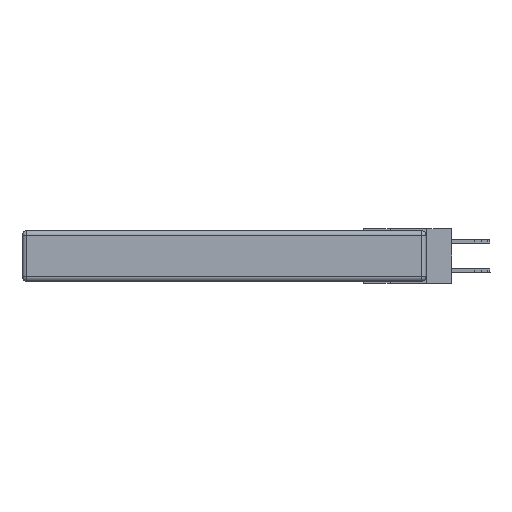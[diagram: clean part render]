
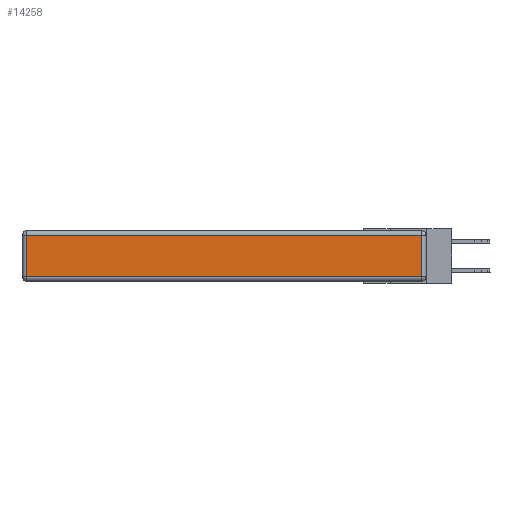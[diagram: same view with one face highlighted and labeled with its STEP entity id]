
A CAD part, left-side view. The second image highlights one B-rep face of the part: STEP entity #14258.
In plain terms, the highlighted planar face has unit normal (-1, 0, 0).
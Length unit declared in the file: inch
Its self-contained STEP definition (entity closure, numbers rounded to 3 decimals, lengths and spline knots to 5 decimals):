
#116 = CARTESIAN_POINT ( 'NONE',  ( 0., 0.03, -0.03 ) ) ;
#505 = DIRECTION ( 'NONE',  ( 0., 0., 1. ) ) ;
#1072 = VECTOR ( 'NONE', #21567, 39.37008 ) ;
#3934 = VECTOR ( 'NONE', #12660, 39.37008 ) ;
#4353 = VERTEX_POINT ( 'NONE', #11014 ) ;
#4392 = VECTOR ( 'NONE', #18803, 39.37008 ) ;
#4540 = VERTEX_POINT ( 'NONE', #116 ) ;
#4921 = CARTESIAN_POINT ( 'NONE',  ( 0., 0., -0.313 ) ) ;
#5658 = LINE ( 'NONE', #12827, #3934 ) ;
#5936 = CARTESIAN_POINT ( 'NONE',  ( 0., 2.72, -0.343 ) ) ;
#6780 = EDGE_CURVE ( 'NONE', #17290, #23085, #12597, .T. ) ;
#6878 = ORIENTED_EDGE ( 'NONE', *, *, #8511, .T. ) ;
#6941 = AXIS2_PLACEMENT_3D ( 'NONE', #7834, #11496, #505 ) ;
#7834 = CARTESIAN_POINT ( 'NONE',  ( 0., 0., -0.343 ) ) ;
#8511 = EDGE_CURVE ( 'NONE', #4540, #4353, #15452, .T. ) ;
#10139 = LINE ( 'NONE', #5936, #4392 ) ;
#10734 = CARTESIAN_POINT ( 'NONE',  ( 0., 2.75, -0.03 ) ) ;
#11014 = CARTESIAN_POINT ( 'NONE',  ( 0., 2.72, -0.03 ) ) ;
#11496 = DIRECTION ( 'NONE',  ( -1., 0., 0. ) ) ;
#12597 = LINE ( 'NONE', #4921, #21541 ) ;
#12660 = DIRECTION ( 'NONE',  ( 0., 0., 1. ) ) ;
#12827 = CARTESIAN_POINT ( 'NONE',  ( 0., 0.03, -0.343 ) ) ;
#13038 = ORIENTED_EDGE ( 'NONE', *, *, #6780, .T. ) ;
#13878 = EDGE_LOOP ( 'NONE', ( #13038, #23063, #6878, #19688 ) ) ;
#14258 = ADVANCED_FACE ( 'NONE', ( #17523 ), #22600, .T. ) ;
#15261 = CARTESIAN_POINT ( 'NONE',  ( 0., 2.72, -0.313 ) ) ;
#15452 = LINE ( 'NONE', #10734, #1072 ) ;
#17290 = VERTEX_POINT ( 'NONE', #15261 ) ;
#17523 = FACE_OUTER_BOUND ( 'NONE', #13878, .T. ) ;
#17780 = DIRECTION ( 'NONE',  ( 0., -1., 0. ) ) ;
#18783 = EDGE_CURVE ( 'NONE', #4353, #17290, #10139, .T. ) ;
#18803 = DIRECTION ( 'NONE',  ( 0., 0., -1. ) ) ;
#19688 = ORIENTED_EDGE ( 'NONE', *, *, #18783, .T. ) ;
#21541 = VECTOR ( 'NONE', #17780, 39.37008 ) ;
#21567 = DIRECTION ( 'NONE',  ( 0., 1., 0. ) ) ;
#22600 = PLANE ( 'NONE',  #6941 ) ;
#22813 = EDGE_CURVE ( 'NONE', #23085, #4540, #5658, .T. ) ;
#23063 = ORIENTED_EDGE ( 'NONE', *, *, #22813, .T. ) ;
#23085 = VERTEX_POINT ( 'NONE', #23597 ) ;
#23597 = CARTESIAN_POINT ( 'NONE',  ( 0., 0.03, -0.313 ) ) ;
